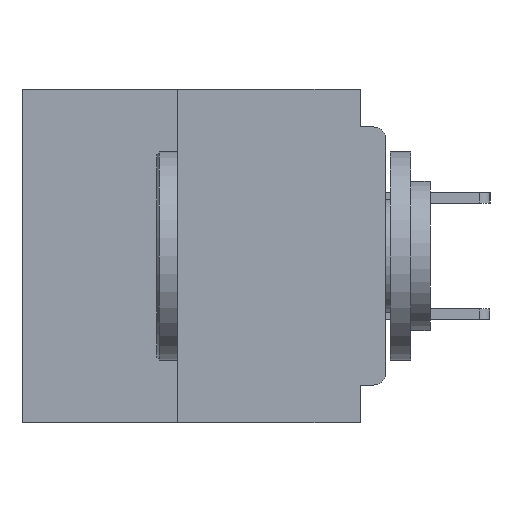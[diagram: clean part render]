
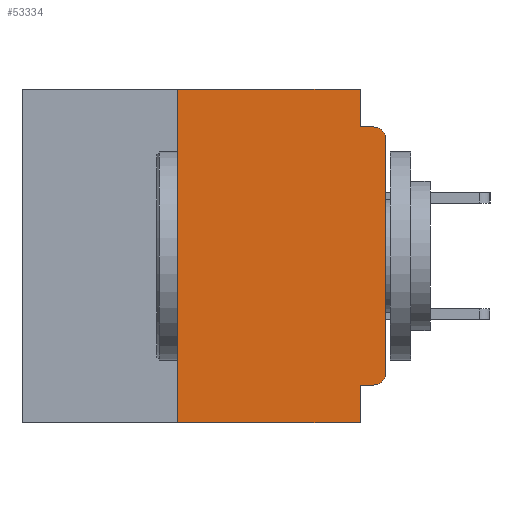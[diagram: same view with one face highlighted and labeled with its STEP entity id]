
A CAD part, left-side view. The second image highlights one B-rep face of the part: STEP entity #53334.
In plain terms, the highlighted planar face has unit normal (-1, 0, 0).
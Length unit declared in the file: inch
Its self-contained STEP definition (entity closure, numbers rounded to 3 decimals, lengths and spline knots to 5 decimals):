
#790 = CARTESIAN_POINT ( 'NONE',  ( 0., 0., 0. ) ) ;
#921 = VECTOR ( 'NONE', #3637, 39.37008 ) ;
#963 = EDGE_CURVE ( 'NONE', #50091, #18693, #12591, .T. ) ;
#1181 = VERTEX_POINT ( 'NONE', #50377 ) ;
#1735 = EDGE_CURVE ( 'NONE', #39979, #1181, #14050, .T. ) ;
#1969 = ORIENTED_EDGE ( 'NONE', *, *, #1735, .F. ) ;
#2032 = EDGE_LOOP ( 'NONE', ( #25619, #35330, #1969, #46789, #15229, #19416, #9963, #31547, #30601, #23859 ) ) ;
#2342 = CARTESIAN_POINT ( 'NONE',  ( 0., 0.015, -0.355 ) ) ;
#2481 = CARTESIAN_POINT ( 'NONE',  ( 0., 0.437, 0. ) ) ;
#3464 = DIRECTION ( 'NONE',  ( 0., -1., 0. ) ) ;
#3637 = DIRECTION ( 'NONE',  ( 0., -1., 0. ) ) ;
#3843 = CARTESIAN_POINT ( 'NONE',  ( 0., 0., -0.045 ) ) ;
#4745 = LINE ( 'NONE', #55706, #29404 ) ;
#7285 = EDGE_CURVE ( 'NONE', #18693, #33416, #26313, .T. ) ;
#7573 = DIRECTION ( 'NONE',  ( 0., 0., -1. ) ) ;
#7587 = EDGE_CURVE ( 'NONE', #49061, #9007, #22436, .T. ) ;
#8602 = EDGE_CURVE ( 'NONE', #18216, #1181, #40732, .T. ) ;
#9007 = VERTEX_POINT ( 'NONE', #20353 ) ;
#9963 = ORIENTED_EDGE ( 'NONE', *, *, #51499, .T. ) ;
#10688 = DIRECTION ( 'NONE',  ( 0., 0., 1. ) ) ;
#10826 = VECTOR ( 'NONE', #36933, 39.37008 ) ;
#11044 = VECTOR ( 'NONE', #13399, 39.37008 ) ;
#11514 = CIRCLE ( 'NONE', #59795, 0.015 ) ;
#12591 = LINE ( 'NONE', #13098, #11044 ) ;
#13098 = CARTESIAN_POINT ( 'NONE',  ( 0., 0., -0.355 ) ) ;
#13399 = DIRECTION ( 'NONE',  ( 0., 1., 0. ) ) ;
#14050 = LINE ( 'NONE', #3843, #921 ) ;
#15229 = ORIENTED_EDGE ( 'NONE', *, *, #7587, .F. ) ;
#18031 = EDGE_CURVE ( 'NONE', #28275, #49061, #4745, .T. ) ;
#18216 = VERTEX_POINT ( 'NONE', #52037 ) ;
#18693 = VERTEX_POINT ( 'NONE', #21293 ) ;
#19416 = ORIENTED_EDGE ( 'NONE', *, *, #18031, .F. ) ;
#20192 = DIRECTION ( 'NONE',  ( -1., 0., 0. ) ) ;
#20353 = CARTESIAN_POINT ( 'NONE',  ( 0., 0.031, 0. ) ) ;
#21293 = CARTESIAN_POINT ( 'NONE',  ( 0., 0.031, -0.355 ) ) ;
#22436 = LINE ( 'NONE', #2481, #10826 ) ;
#23859 = ORIENTED_EDGE ( 'NONE', *, *, #62426, .T. ) ;
#24814 = CARTESIAN_POINT ( 'NONE',  ( 0., 0.031, -0.045 ) ) ;
#24832 = CARTESIAN_POINT ( 'NONE',  ( 0., 0.25, -0.4 ) ) ;
#25619 = ORIENTED_EDGE ( 'NONE', *, *, #40679, .T. ) ;
#25809 = CARTESIAN_POINT ( 'NONE',  ( 0., 0., -0.34 ) ) ;
#26105 = CARTESIAN_POINT ( 'NONE',  ( 0., 0.015, -0.06 ) ) ;
#26313 = LINE ( 'NONE', #59296, #40913 ) ;
#26365 = CARTESIAN_POINT ( 'NONE',  ( 0., 0.437, 0. ) ) ;
#26392 = FACE_OUTER_BOUND ( 'NONE', #2032, .T. ) ;
#27000 = LINE ( 'NONE', #32099, #38531 ) ;
#27441 = VECTOR ( 'NONE', #10688, 39.37008 ) ;
#28275 = VERTEX_POINT ( 'NONE', #24832 ) ;
#29404 = VECTOR ( 'NONE', #60621, 39.37008 ) ;
#29805 = AXIS2_PLACEMENT_3D ( 'NONE', #26365, #60671, #31291 ) ;
#29900 = DIRECTION ( 'NONE',  ( 0., 0., -1. ) ) ;
#30601 = ORIENTED_EDGE ( 'NONE', *, *, #963, .F. ) ;
#31031 = DIRECTION ( 'NONE',  ( 0., 0., -1. ) ) ;
#31291 = DIRECTION ( 'NONE',  ( 0., 0., -1. ) ) ;
#31547 = ORIENTED_EDGE ( 'NONE', *, *, #7285, .F. ) ;
#32099 = CARTESIAN_POINT ( 'NONE',  ( 0., 0.031, 0. ) ) ;
#33416 = VERTEX_POINT ( 'NONE', #61163 ) ;
#35330 = ORIENTED_EDGE ( 'NONE', *, *, #8602, .T. ) ;
#36933 = DIRECTION ( 'NONE',  ( 0., -1., 0. ) ) ;
#38531 = VECTOR ( 'NONE', #7573, 39.37008 ) ;
#39979 = VERTEX_POINT ( 'NONE', #24814 ) ;
#40377 = LINE ( 'NONE', #52501, #51849 ) ;
#40679 = EDGE_CURVE ( 'NONE', #52583, #18216, #53544, .T. ) ;
#40732 = CIRCLE ( 'NONE', #55326, 0.015 ) ;
#40913 = VECTOR ( 'NONE', #29900, 39.37008 ) ;
#45684 = CARTESIAN_POINT ( 'NONE',  ( 0., 0.25, 0. ) ) ;
#46789 = ORIENTED_EDGE ( 'NONE', *, *, #61501, .F. ) ;
#49061 = VERTEX_POINT ( 'NONE', #45684 ) ;
#49589 = CARTESIAN_POINT ( 'NONE',  ( 0., 0.015, -0.34 ) ) ;
#50091 = VERTEX_POINT ( 'NONE', #2342 ) ;
#50377 = CARTESIAN_POINT ( 'NONE',  ( 0., 0.015, -0.045 ) ) ;
#51499 = EDGE_CURVE ( 'NONE', #28275, #33416, #40377, .T. ) ;
#51849 = VECTOR ( 'NONE', #3464, 39.37008 ) ;
#52037 = CARTESIAN_POINT ( 'NONE',  ( 0., 0., -0.06 ) ) ;
#52501 = CARTESIAN_POINT ( 'NONE',  ( 0., 0.437, -0.4 ) ) ;
#52583 = VERTEX_POINT ( 'NONE', #25809 ) ;
#53334 = ADVANCED_FACE ( 'NONE', ( #26392 ), #55761, .F. ) ;
#53544 = LINE ( 'NONE', #790, #27441 ) ;
#54541 = DIRECTION ( 'NONE',  ( 0., 0., -1. ) ) ;
#55326 = AXIS2_PLACEMENT_3D ( 'NONE', #26105, #60416, #31031 ) ;
#55706 = CARTESIAN_POINT ( 'NONE',  ( 0., 0.25, -0.4 ) ) ;
#55761 = PLANE ( 'NONE',  #29805 ) ;
#59296 = CARTESIAN_POINT ( 'NONE',  ( 0., 0.031, -0.4 ) ) ;
#59795 = AXIS2_PLACEMENT_3D ( 'NONE', #49589, #20192, #54541 ) ;
#60416 = DIRECTION ( 'NONE',  ( -1., 0., 0. ) ) ;
#60621 = DIRECTION ( 'NONE',  ( 0., 0., 1. ) ) ;
#60671 = DIRECTION ( 'NONE',  ( 1., 0., 0. ) ) ;
#61163 = CARTESIAN_POINT ( 'NONE',  ( 0., 0.031, -0.4 ) ) ;
#61501 = EDGE_CURVE ( 'NONE', #9007, #39979, #27000, .T. ) ;
#62426 = EDGE_CURVE ( 'NONE', #50091, #52583, #11514, .T. ) ;
